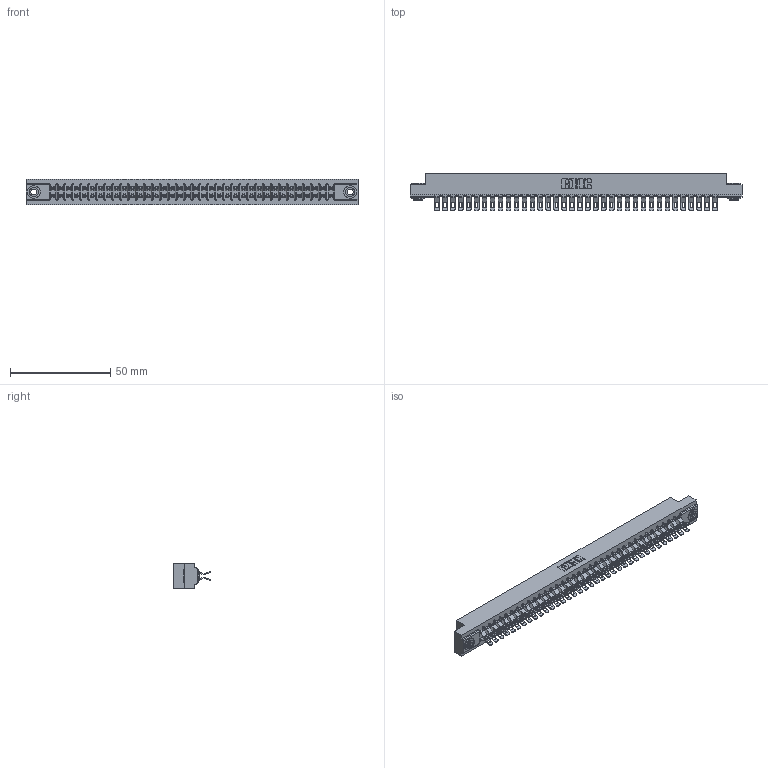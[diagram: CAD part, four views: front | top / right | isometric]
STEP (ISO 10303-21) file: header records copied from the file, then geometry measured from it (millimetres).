
FILE_DESCRIPTION (( 'STEP AP203' ), '1' );
FILE_NAME ('357-072-455-203.STEP', '2020-10-04T19:29:17', ( '' ), ( '' ), 'SwSTEP 2.0', 'SolidWorks 2020', '' );
FILE_SCHEMA (( 'CONFIG_CONTROL_DESIGN' ));
Length unit declared in the file: inch
Products named in the file (4): 357-072-455-203; 307 Part_.156 Dia Mounting Holes; 345-250-002_345-250-002-102; 307-290-001_555
Assembly tree (75 placements, depth 2):
  357-072-455-203
    307 Part_.156 Dia Mounting Holes
    307-290-001_555  x72
    345-250-002_345-250-002-102  x2
Bounding box: 165.66 x 18.75 x 12.7 mm (x, y, z)
Volume: 17789.2 mm3; surface area: 23086.1 mm2
Topology: 75 solids, 75 shells, 4599 faces, 13467 edges, 8778 vertices
Faces by surface type: plane 2542, cylinder 1975, sphere 74, cone 8
Entity records: 34356 total; most frequent: CARTESIAN_POINT 5609, ORIENTED_EDGE 5552, DIRECTION 5518, EDGE_CURVE 2776, LINE 2108, VECTOR 2108, VERTEX_POINT 1796, AXIS2_PLACEMENT_3D 1705
